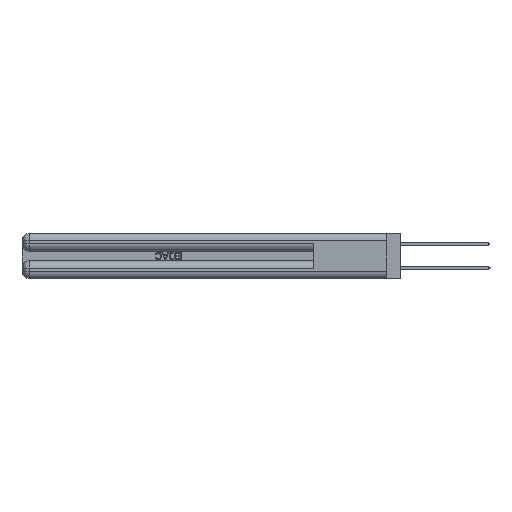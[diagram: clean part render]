
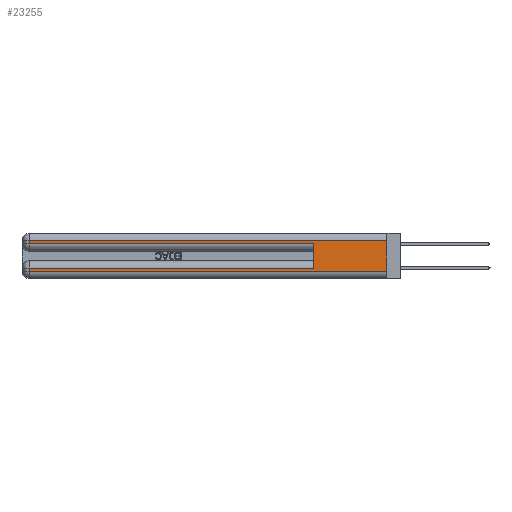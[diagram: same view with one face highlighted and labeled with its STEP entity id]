
A CAD part, left-side view. The second image highlights one B-rep face of the part: STEP entity #23255.
In plain terms, the highlighted planar face has unit normal (-1, 0, 0).
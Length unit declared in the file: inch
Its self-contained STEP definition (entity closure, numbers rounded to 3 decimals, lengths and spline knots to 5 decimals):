
#154 = EDGE_CURVE ( 'NONE', #31294, #14360, #26794, .T. ) ;
#1274 = ORIENTED_EDGE ( 'NONE', *, *, #27955, .T. ) ;
#1320 = DIRECTION ( 'NONE',  ( 0., 0., -1. ) ) ;
#1451 = LINE ( 'NONE', #27066, #4285 ) ;
#2107 = VECTOR ( 'NONE', #15131, 39.37008 ) ;
#2740 = VERTEX_POINT ( 'NONE', #17781 ) ;
#2840 = LINE ( 'NONE', #31439, #14371 ) ;
#3794 = EDGE_CURVE ( 'NONE', #16486, #28154, #22398, .T. ) ;
#4285 = VECTOR ( 'NONE', #15526, 39.37008 ) ;
#9242 = CARTESIAN_POINT ( 'NONE',  ( 0., 0., 0.06 ) ) ;
#11154 = DIRECTION ( 'NONE',  ( 0., 1., 0. ) ) ;
#11558 = VERTEX_POINT ( 'NONE', #43732 ) ;
#12220 = EDGE_LOOP ( 'NONE', ( #15366, #1274, #31007, #33921, #30565, #16715, #12372, #33351 ) ) ;
#12372 = ORIENTED_EDGE ( 'NONE', *, *, #46675, .T. ) ;
#12477 = CARTESIAN_POINT ( 'NONE',  ( 0., 2.94, 0.37 ) ) ;
#13679 = EDGE_CURVE ( 'NONE', #29342, #28154, #2840, .T. ) ;
#14170 = EDGE_CURVE ( 'NONE', #11558, #2740, #34281, .T. ) ;
#14360 = VERTEX_POINT ( 'NONE', #31019 ) ;
#14371 = VECTOR ( 'NONE', #20444, 39.37008 ) ;
#14597 = VECTOR ( 'NONE', #45808, 39.37008 ) ;
#15076 = DIRECTION ( 'NONE',  ( 0., -1., 0. ) ) ;
#15131 = DIRECTION ( 'NONE',  ( 0., -1., 0. ) ) ;
#15366 = ORIENTED_EDGE ( 'NONE', *, *, #13679, .F. ) ;
#15526 = DIRECTION ( 'NONE',  ( 0., 0., 1. ) ) ;
#16486 = VERTEX_POINT ( 'NONE', #43234 ) ;
#16715 = ORIENTED_EDGE ( 'NONE', *, *, #14170, .T. ) ;
#17781 = CARTESIAN_POINT ( 'NONE',  ( 0., 2.94, 0.085 ) ) ;
#18959 = VECTOR ( 'NONE', #46072, 39.37008 ) ;
#20067 = PLANE ( 'NONE',  #30346 ) ;
#20215 = DIRECTION ( 'NONE',  ( 1., 0., 0. ) ) ;
#20444 = DIRECTION ( 'NONE',  ( 0., 0., -1. ) ) ;
#20624 = EDGE_CURVE ( 'NONE', #11558, #14360, #1451, .T. ) ;
#22398 = LINE ( 'NONE', #33881, #28131 ) ;
#22561 = VERTEX_POINT ( 'NONE', #31996 ) ;
#23255 = ADVANCED_FACE ( 'NONE', ( #43657 ), #20067, .F. ) ;
#24480 = LINE ( 'NONE', #33103, #36989 ) ;
#24495 = CARTESIAN_POINT ( 'NONE',  ( 0., 0., 0.31 ) ) ;
#26794 = LINE ( 'NONE', #40371, #2107 ) ;
#27066 = CARTESIAN_POINT ( 'NONE',  ( 0., 0.6, 0.145 ) ) ;
#27090 = DIRECTION ( 'NONE',  ( 0., 0., -1. ) ) ;
#27955 = EDGE_CURVE ( 'NONE', #29342, #22561, #24480, .T. ) ;
#28131 = VECTOR ( 'NONE', #15076, 39.37008 ) ;
#28154 = VERTEX_POINT ( 'NONE', #9242 ) ;
#29342 = VERTEX_POINT ( 'NONE', #24495 ) ;
#30346 = AXIS2_PLACEMENT_3D ( 'NONE', #42000, #20215, #1320 ) ;
#30565 = ORIENTED_EDGE ( 'NONE', *, *, #20624, .F. ) ;
#31007 = ORIENTED_EDGE ( 'NONE', *, *, #38587, .T. ) ;
#31019 = CARTESIAN_POINT ( 'NONE',  ( 0., 0.6, 0.285 ) ) ;
#31294 = VERTEX_POINT ( 'NONE', #42771 ) ;
#31439 = CARTESIAN_POINT ( 'NONE',  ( 0., 0., 0.37 ) ) ;
#31996 = CARTESIAN_POINT ( 'NONE',  ( 0., 2.94, 0.31 ) ) ;
#33103 = CARTESIAN_POINT ( 'NONE',  ( 0., 0., 0.31 ) ) ;
#33351 = ORIENTED_EDGE ( 'NONE', *, *, #3794, .T. ) ;
#33881 = CARTESIAN_POINT ( 'NONE',  ( 0., 0., 0.06 ) ) ;
#33921 = ORIENTED_EDGE ( 'NONE', *, *, #154, .T. ) ;
#34281 = LINE ( 'NONE', #41227, #18959 ) ;
#36989 = VECTOR ( 'NONE', #11154, 39.37008 ) ;
#38587 = EDGE_CURVE ( 'NONE', #22561, #31294, #43199, .T. ) ;
#40371 = CARTESIAN_POINT ( 'NONE',  ( 0., 0., 0.285 ) ) ;
#41227 = CARTESIAN_POINT ( 'NONE',  ( 0., 0., 0.085 ) ) ;
#42000 = CARTESIAN_POINT ( 'NONE',  ( 0., 0., 0.37 ) ) ;
#42395 = CARTESIAN_POINT ( 'NONE',  ( 0., 2.94, 0.37 ) ) ;
#42771 = CARTESIAN_POINT ( 'NONE',  ( 0., 2.94, 0.285 ) ) ;
#43199 = LINE ( 'NONE', #42395, #14597 ) ;
#43234 = CARTESIAN_POINT ( 'NONE',  ( 0., 2.94, 0.06 ) ) ;
#43657 = FACE_OUTER_BOUND ( 'NONE', #12220, .T. ) ;
#43732 = CARTESIAN_POINT ( 'NONE',  ( 0., 0.6, 0.085 ) ) ;
#44815 = LINE ( 'NONE', #12477, #47146 ) ;
#45808 = DIRECTION ( 'NONE',  ( 0., 0., -1. ) ) ;
#46072 = DIRECTION ( 'NONE',  ( 0., 1., 0. ) ) ;
#46675 = EDGE_CURVE ( 'NONE', #2740, #16486, #44815, .T. ) ;
#47146 = VECTOR ( 'NONE', #27090, 39.37008 ) ;
